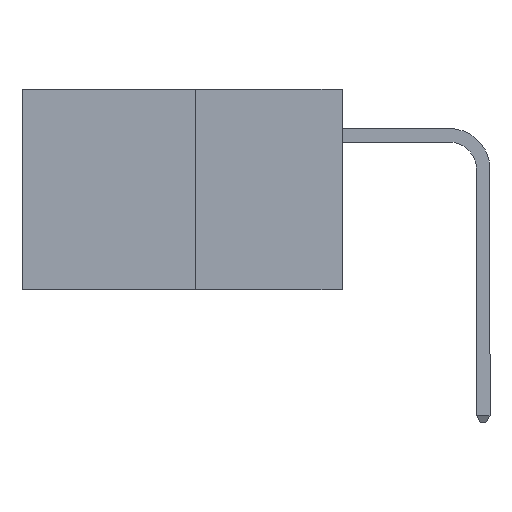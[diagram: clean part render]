
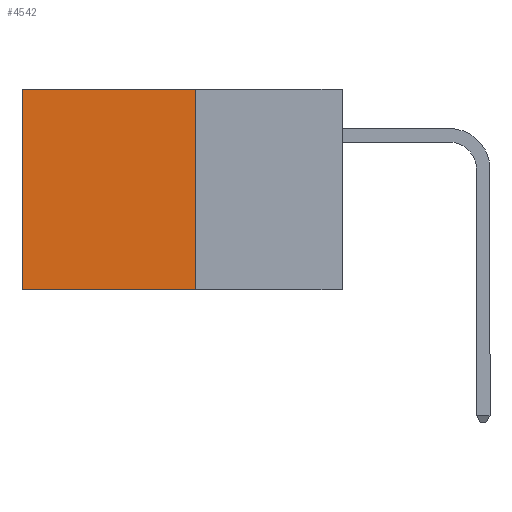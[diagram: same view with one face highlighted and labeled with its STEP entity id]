
A CAD part, left-side view. The second image highlights one B-rep face of the part: STEP entity #4542.
In plain terms, the highlighted planar face has unit normal (-1, 0, 0).
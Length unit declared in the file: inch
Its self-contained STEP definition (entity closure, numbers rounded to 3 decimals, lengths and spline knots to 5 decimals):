
#73 = VERTEX_POINT ( 'NONE', #8269 ) ;
#739 = CARTESIAN_POINT ( 'NONE',  ( 0.277, 0.59, 0. ) ) ;
#882 = VERTEX_POINT ( 'NONE', #8501 ) ;
#1119 = DIRECTION ( 'NONE',  ( 0., 0., -1. ) ) ;
#1232 = CARTESIAN_POINT ( 'NONE',  ( 0.277, 0.27, -0.37 ) ) ;
#1415 = CARTESIAN_POINT ( 'NONE',  ( 0.277, 0.27, -0.37 ) ) ;
#1526 = DIRECTION ( 'NONE',  ( 1., 0., 0. ) ) ;
#1579 = LINE ( 'NONE', #2000, #8747 ) ;
#1886 = EDGE_CURVE ( 'NONE', #6046, #4909, #3178, .T. ) ;
#2000 = CARTESIAN_POINT ( 'NONE',  ( 0.277, 0.59, -0.37 ) ) ;
#2162 = DIRECTION ( 'NONE',  ( 0., 0., -1. ) ) ;
#2618 = FACE_OUTER_BOUND ( 'NONE', #4926, .T. ) ;
#2834 = ORIENTED_EDGE ( 'NONE', *, *, #4913, .T. ) ;
#2875 = ORIENTED_EDGE ( 'NONE', *, *, #5633, .F. ) ;
#2938 = ORIENTED_EDGE ( 'NONE', *, *, #5264, .F. ) ;
#2966 = LINE ( 'NONE', #4941, #6616 ) ;
#2979 = ORIENTED_EDGE ( 'NONE', *, *, #1886, .T. ) ;
#3178 = LINE ( 'NONE', #6082, #8403 ) ;
#3787 = CARTESIAN_POINT ( 'NONE',  ( 0.277, 0.27, 0. ) ) ;
#3792 = DIRECTION ( 'NONE',  ( 0., 1., 0. ) ) ;
#4111 = PLANE ( 'NONE',  #4167 ) ;
#4167 = AXIS2_PLACEMENT_3D ( 'NONE', #1415, #1526, #6412 ) ;
#4198 = LINE ( 'NONE', #1232, #6224 ) ;
#4542 = ADVANCED_FACE ( 'NONE', ( #2618 ), #4111, .F. ) ;
#4909 = VERTEX_POINT ( 'NONE', #739 ) ;
#4913 = EDGE_CURVE ( 'NONE', #4909, #73, #1579, .T. ) ;
#4926 = EDGE_LOOP ( 'NONE', ( #2834, #2875, #2938, #2979 ) ) ;
#4941 = CARTESIAN_POINT ( 'NONE',  ( 0.277, 0.27, -0.37 ) ) ;
#5228 = DIRECTION ( 'NONE',  ( 0., 1., 0. ) ) ;
#5264 = EDGE_CURVE ( 'NONE', #6046, #882, #4198, .T. ) ;
#5633 = EDGE_CURVE ( 'NONE', #882, #73, #2966, .T. ) ;
#6046 = VERTEX_POINT ( 'NONE', #3787 ) ;
#6082 = CARTESIAN_POINT ( 'NONE',  ( 0.277, 0.27, 0. ) ) ;
#6224 = VECTOR ( 'NONE', #1119, 39.37008 ) ;
#6412 = DIRECTION ( 'NONE',  ( 0., 0., -1. ) ) ;
#6616 = VECTOR ( 'NONE', #5228, 39.37008 ) ;
#8269 = CARTESIAN_POINT ( 'NONE',  ( 0.277, 0.59, -0.37 ) ) ;
#8403 = VECTOR ( 'NONE', #3792, 39.37008 ) ;
#8501 = CARTESIAN_POINT ( 'NONE',  ( 0.277, 0.27, -0.37 ) ) ;
#8747 = VECTOR ( 'NONE', #2162, 39.37008 ) ;
